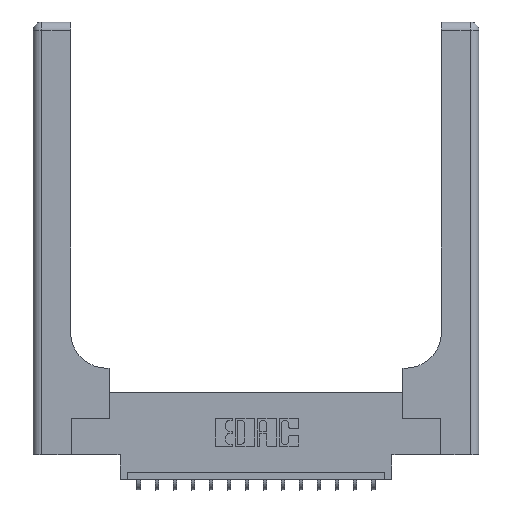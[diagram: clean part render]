
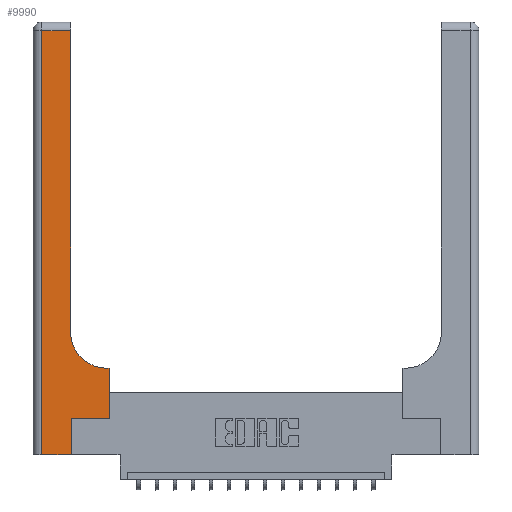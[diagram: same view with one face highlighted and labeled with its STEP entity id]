
A CAD part, top view. The second image highlights one B-rep face of the part: STEP entity #9990.
In plain terms, the highlighted planar face has unit normal (0, 0, 1).
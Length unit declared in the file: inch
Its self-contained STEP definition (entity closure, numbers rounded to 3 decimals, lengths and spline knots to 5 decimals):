
#324 = DIRECTION ( 'NONE',  ( 0., 0., -1. ) ) ;
#368 = CARTESIAN_POINT ( 'NONE',  ( 0.06, 3., 0.37 ) ) ;
#876 = ORIENTED_EDGE ( 'NONE', *, *, #7840, .T. ) ;
#941 = CARTESIAN_POINT ( 'NONE',  ( 0.26, 0.6, 0.37 ) ) ;
#1167 = CARTESIAN_POINT ( 'NONE',  ( 0.528, 0.25, 0.37 ) ) ;
#1174 = ORIENTED_EDGE ( 'NONE', *, *, #5857, .T. ) ;
#1208 = EDGE_CURVE ( 'NONE', #12133, #1992, #8382, .T. ) ;
#1306 = ORIENTED_EDGE ( 'NONE', *, *, #6783, .T. ) ;
#1362 = ORIENTED_EDGE ( 'NONE', *, *, #1208, .T. ) ;
#1445 = CARTESIAN_POINT ( 'NONE',  ( 0.265, 0.25, 0.37 ) ) ;
#1733 = VERTEX_POINT ( 'NONE', #8827 ) ;
#1808 = EDGE_CURVE ( 'NONE', #1992, #1733, #10297, .T. ) ;
#1829 = CARTESIAN_POINT ( 'NONE',  ( 0.26, 3., 0.37 ) ) ;
#1906 = LINE ( 'NONE', #1829, #5610 ) ;
#1992 = VERTEX_POINT ( 'NONE', #1167 ) ;
#2183 = AXIS2_PLACEMENT_3D ( 'NONE', #8628, #324, #10012 ) ;
#2240 = DIRECTION ( 'NONE',  ( 0., 0., -1. ) ) ;
#2306 = VERTEX_POINT ( 'NONE', #17380 ) ;
#2566 = DIRECTION ( 'NONE',  ( -1., 0., 0. ) ) ;
#3410 = VECTOR ( 'NONE', #9536, 39.37008 ) ;
#3718 = FACE_OUTER_BOUND ( 'NONE', #12733, .T. ) ;
#4147 = CARTESIAN_POINT ( 'NONE',  ( 0.265, 0.25, 0.37 ) ) ;
#4389 = VERTEX_POINT ( 'NONE', #9623 ) ;
#4678 = VECTOR ( 'NONE', #9091, 39.37008 ) ;
#5062 = DIRECTION ( 'NONE',  ( 0., 1., 0. ) ) ;
#5346 = CARTESIAN_POINT ( 'NONE',  ( 0.06, 2.94, 0.37 ) ) ;
#5610 = VECTOR ( 'NONE', #15640, 39.37008 ) ;
#5857 = EDGE_CURVE ( 'NONE', #1733, #7355, #9397, .T. ) ;
#6222 = CARTESIAN_POINT ( 'NONE',  ( 0.528, 0.25, 0.37 ) ) ;
#6405 = CARTESIAN_POINT ( 'NONE',  ( 0.265, 0., 0.37 ) ) ;
#6473 = DIRECTION ( 'NONE',  ( -1., 0., 0. ) ) ;
#6608 = VECTOR ( 'NONE', #10391, 39.37008 ) ;
#6783 = EDGE_CURVE ( 'NONE', #17119, #9798, #13671, .T. ) ;
#7235 = CARTESIAN_POINT ( 'NONE',  ( 0.265, 0., 0.37 ) ) ;
#7238 = ORIENTED_EDGE ( 'NONE', *, *, #1808, .T. ) ;
#7355 = VERTEX_POINT ( 'NONE', #15371 ) ;
#7766 = ORIENTED_EDGE ( 'NONE', *, *, #17199, .T. ) ;
#7840 = EDGE_CURVE ( 'NONE', #2306, #17119, #13215, .T. ) ;
#8126 = CARTESIAN_POINT ( 'NONE',  ( 0., 2.94, 0.37 ) ) ;
#8382 = LINE ( 'NONE', #4147, #4678 ) ;
#8628 = CARTESIAN_POINT ( 'NONE',  ( 0.51, 0.85, 0.37 ) ) ;
#8827 = CARTESIAN_POINT ( 'NONE',  ( 0.528, 0.6, 0.37 ) ) ;
#9091 = DIRECTION ( 'NONE',  ( 1., 0., 0. ) ) ;
#9397 = LINE ( 'NONE', #941, #16680 ) ;
#9536 = DIRECTION ( 'NONE',  ( 1., 0., 0. ) ) ;
#9602 = EDGE_CURVE ( 'NONE', #9798, #9811, #10793, .T. ) ;
#9623 = CARTESIAN_POINT ( 'NONE',  ( 0.26, 0.85, 0.37 ) ) ;
#9798 = VERTEX_POINT ( 'NONE', #16709 ) ;
#9811 = VERTEX_POINT ( 'NONE', #7235 ) ;
#9990 = ADVANCED_FACE ( 'NONE', ( #3718 ), #14606, .F. ) ;
#10012 = DIRECTION ( 'NONE',  ( 1., 0., 0. ) ) ;
#10048 = VECTOR ( 'NONE', #15560, 39.37008 ) ;
#10297 = LINE ( 'NONE', #6222, #6608 ) ;
#10391 = DIRECTION ( 'NONE',  ( 0., 1., 0. ) ) ;
#10548 = CARTESIAN_POINT ( 'NONE',  ( 0., 3., 0.37 ) ) ;
#10793 = LINE ( 'NONE', #17685, #3410 ) ;
#11277 = ORIENTED_EDGE ( 'NONE', *, *, #9602, .T. ) ;
#11910 = DIRECTION ( 'NONE',  ( -1., 0., 0. ) ) ;
#11916 = VECTOR ( 'NONE', #2566, 39.37008 ) ;
#12133 = VERTEX_POINT ( 'NONE', #1445 ) ;
#12148 = ORIENTED_EDGE ( 'NONE', *, *, #14176, .T. ) ;
#12733 = EDGE_LOOP ( 'NONE', ( #17073, #876, #1306, #11277, #12148, #1362, #7238, #1174, #7766 ) ) ;
#12980 = EDGE_CURVE ( 'NONE', #4389, #2306, #1906, .T. ) ;
#13215 = LINE ( 'NONE', #8126, #11916 ) ;
#13671 = LINE ( 'NONE', #368, #10048 ) ;
#14162 = VECTOR ( 'NONE', #5062, 39.37008 ) ;
#14176 = EDGE_CURVE ( 'NONE', #9811, #12133, #17822, .T. ) ;
#14606 = PLANE ( 'NONE',  #15054 ) ;
#15054 = AXIS2_PLACEMENT_3D ( 'NONE', #10548, #2240, #11910 ) ;
#15371 = CARTESIAN_POINT ( 'NONE',  ( 0.51, 0.6, 0.37 ) ) ;
#15560 = DIRECTION ( 'NONE',  ( 0., -1., 0. ) ) ;
#15640 = DIRECTION ( 'NONE',  ( 0., 1., 0. ) ) ;
#16680 = VECTOR ( 'NONE', #6473, 39.37008 ) ;
#16709 = CARTESIAN_POINT ( 'NONE',  ( 0.06, 0., 0.37 ) ) ;
#17073 = ORIENTED_EDGE ( 'NONE', *, *, #12980, .T. ) ;
#17119 = VERTEX_POINT ( 'NONE', #5346 ) ;
#17199 = EDGE_CURVE ( 'NONE', #7355, #4389, #17413, .T. ) ;
#17380 = CARTESIAN_POINT ( 'NONE',  ( 0.26, 2.94, 0.37 ) ) ;
#17413 = CIRCLE ( 'NONE', #2183, 0.25 ) ;
#17685 = CARTESIAN_POINT ( 'NONE',  ( 0., 0., 0.37 ) ) ;
#17822 = LINE ( 'NONE', #6405, #14162 ) ;
